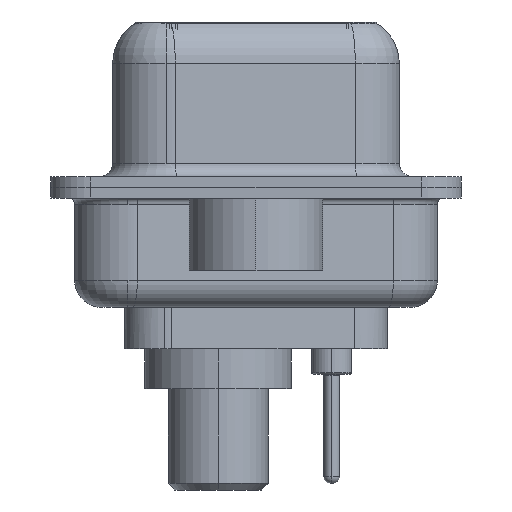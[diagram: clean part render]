
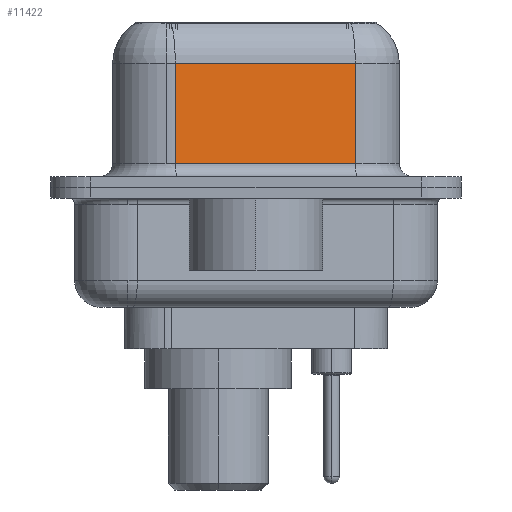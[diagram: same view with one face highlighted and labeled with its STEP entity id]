
A CAD part, left-side view. The second image highlights one B-rep face of the part: STEP entity #11422.
In plain terms, the highlighted planar face has unit normal (-0.985, -0.174, 0).
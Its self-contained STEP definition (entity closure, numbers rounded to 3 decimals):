
#1335 = ORIENTED_EDGE ( 'NONE', *, *, #2488, .T. ) ;
#1622 = VERTEX_POINT ( 'NONE', #31495 ) ;
#2488 = EDGE_CURVE ( 'NONE', #1622, #19659, #11242, .T. ) ;
#3446 = VERTEX_POINT ( 'NONE', #24885 ) ;
#3464 = EDGE_CURVE ( 'NONE', #3446, #1622, #19141, .T. ) ;
#5305 = ORIENTED_EDGE ( 'NONE', *, *, #14648, .T. ) ;
#6026 = LINE ( 'NONE', #8689, #33168 ) ;
#8689 = CARTESIAN_POINT ( 'NONE',  ( 5.621, -3.722, 6.4 ) ) ;
#9184 = DIRECTION ( 'NONE',  ( -0.174, 0.985, 0. ) ) ;
#10575 = DIRECTION ( 'NONE',  ( 0.985, 0.174, 0. ) ) ;
#10757 = LINE ( 'NONE', #22423, #28997 ) ;
#11242 = LINE ( 'NONE', #28505, #11629 ) ;
#11422 = ADVANCED_FACE ( 'NONE', ( #25453 ), #15544, .F. ) ;
#11629 = VECTOR ( 'NONE', #15457, 1000. ) ;
#14648 = EDGE_CURVE ( 'NONE', #19659, #23602, #10757, .T. ) ;
#15067 = VECTOR ( 'NONE', #9184, 1000. ) ;
#15457 = DIRECTION ( 'NONE',  ( 0., 0., -1. ) ) ;
#15544 = PLANE ( 'NONE',  #19996 ) ;
#15620 = ORIENTED_EDGE ( 'NONE', *, *, #3464, .T. ) ;
#15889 = CARTESIAN_POINT ( 'NONE',  ( 5.621, -3.722, 6.4 ) ) ;
#16723 = DIRECTION ( 'NONE',  ( 0., 0., -1. ) ) ;
#16873 = CARTESIAN_POINT ( 'NONE',  ( 5.621, -3.722, 4.65 ) ) ;
#18255 = ORIENTED_EDGE ( 'NONE', *, *, #32175, .F. ) ;
#18581 = EDGE_LOOP ( 'NONE', ( #18255, #15620, #1335, #5305 ) ) ;
#19141 = LINE ( 'NONE', #16873, #15067 ) ;
#19659 = VERTEX_POINT ( 'NONE', #26774 ) ;
#19996 = AXIS2_PLACEMENT_3D ( 'NONE', #15889, #10575, #23593 ) ;
#21681 = CARTESIAN_POINT ( 'NONE',  ( 5.621, -3.722, 0.9 ) ) ;
#22423 = CARTESIAN_POINT ( 'NONE',  ( 5.621, -3.722, 0.9 ) ) ;
#23593 = DIRECTION ( 'NONE',  ( -0.174, 0.985, 0. ) ) ;
#23602 = VERTEX_POINT ( 'NONE', #21681 ) ;
#24885 = CARTESIAN_POINT ( 'NONE',  ( 5.621, -3.722, 4.65 ) ) ;
#25453 = FACE_OUTER_BOUND ( 'NONE', #18581, .T. ) ;
#26774 = CARTESIAN_POINT ( 'NONE',  ( 4.43, 3.028, 0.9 ) ) ;
#28505 = CARTESIAN_POINT ( 'NONE',  ( 4.43, 3.028, 6.4 ) ) ;
#28997 = VECTOR ( 'NONE', #30131, 1000. ) ;
#30131 = DIRECTION ( 'NONE',  ( 0.174, -0.985, 0. ) ) ;
#31495 = CARTESIAN_POINT ( 'NONE',  ( 4.43, 3.028, 4.65 ) ) ;
#32175 = EDGE_CURVE ( 'NONE', #3446, #23602, #6026, .T. ) ;
#33168 = VECTOR ( 'NONE', #16723, 1000. ) ;
